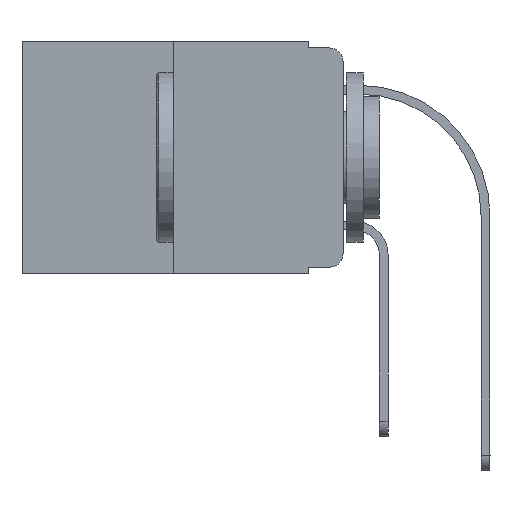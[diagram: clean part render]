
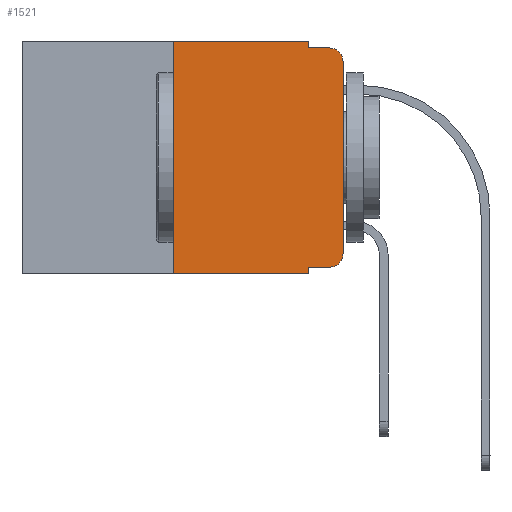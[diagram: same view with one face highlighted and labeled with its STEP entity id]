
A CAD part, left-side view. The second image highlights one B-rep face of the part: STEP entity #1521.
In plain terms, the highlighted planar face has unit normal (-1, 0, 0).
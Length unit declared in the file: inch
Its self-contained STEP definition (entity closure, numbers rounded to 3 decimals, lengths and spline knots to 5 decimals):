
#127 = ORIENTED_EDGE ( 'NONE', *, *, #3472, .F. ) ;
#410 = CARTESIAN_POINT ( 'NONE',  ( 0., 0.02, -0.313 ) ) ;
#486 = DIRECTION ( 'NONE',  ( 0., -1., 0. ) ) ;
#1039 = DIRECTION ( 'NONE',  ( 0., 0., 1. ) ) ;
#1069 = FACE_OUTER_BOUND ( 'NONE', #11055, .T. ) ;
#1080 = VERTEX_POINT ( 'NONE', #9564 ) ;
#1194 = DIRECTION ( 'NONE',  ( -1., 0., 0. ) ) ;
#1281 = CARTESIAN_POINT ( 'NONE',  ( 0., 0.25, 0. ) ) ;
#1407 = VECTOR ( 'NONE', #5567, 39.37008 ) ;
#1521 = ADVANCED_FACE ( 'NONE', ( #1069 ), #3092, .F. ) ;
#1807 = LINE ( 'NONE', #6082, #6714 ) ;
#1906 = CARTESIAN_POINT ( 'NONE',  ( 0., 0.02, -0.03 ) ) ;
#1920 = EDGE_CURVE ( 'NONE', #1080, #12006, #9822, .T. ) ;
#1961 = LINE ( 'NONE', #6384, #5870 ) ;
#2094 = LINE ( 'NONE', #6367, #11426 ) ;
#2271 = EDGE_CURVE ( 'NONE', #12852, #10443, #3841, .T. ) ;
#2323 = AXIS2_PLACEMENT_3D ( 'NONE', #410, #1194, #7557 ) ;
#2445 = VECTOR ( 'NONE', #7130, 39.37008 ) ;
#2518 = LINE ( 'NONE', #4681, #7609 ) ;
#2528 = CARTESIAN_POINT ( 'NONE',  ( 0., 0.051, 0. ) ) ;
#2994 = VERTEX_POINT ( 'NONE', #9002 ) ;
#3092 = PLANE ( 'NONE',  #12811 ) ;
#3226 = DIRECTION ( 'NONE',  ( -1., 0., 0. ) ) ;
#3443 = CARTESIAN_POINT ( 'NONE',  ( 0., 0.25, -0.343 ) ) ;
#3469 = LINE ( 'NONE', #11109, #1407 ) ;
#3472 = EDGE_CURVE ( 'NONE', #2994, #12006, #2518, .T. ) ;
#3476 = CARTESIAN_POINT ( 'NONE',  ( 0., 0.051, -0.333 ) ) ;
#3478 = ORIENTED_EDGE ( 'NONE', *, *, #9224, .F. ) ;
#3704 = CARTESIAN_POINT ( 'NONE',  ( 0., 0.051, -0.333 ) ) ;
#3841 = LINE ( 'NONE', #3704, #2445 ) ;
#3939 = CARTESIAN_POINT ( 'NONE',  ( 0., 0.051, 0. ) ) ;
#4446 = VERTEX_POINT ( 'NONE', #8286 ) ;
#4681 = CARTESIAN_POINT ( 'NONE',  ( 0., 0.051, -0.01 ) ) ;
#5018 = EDGE_CURVE ( 'NONE', #6952, #1080, #1961, .T. ) ;
#5145 = ORIENTED_EDGE ( 'NONE', *, *, #5708, .F. ) ;
#5567 = DIRECTION ( 'NONE',  ( 0., -1., 0. ) ) ;
#5659 = EDGE_CURVE ( 'NONE', #13784, #4446, #3469, .T. ) ;
#5668 = ORIENTED_EDGE ( 'NONE', *, *, #7876, .T. ) ;
#5708 = EDGE_CURVE ( 'NONE', #6629, #2994, #7042, .T. ) ;
#5870 = VECTOR ( 'NONE', #6236, 39.37008 ) ;
#5948 = DIRECTION ( 'NONE',  ( 0., -1., 0. ) ) ;
#5952 = CARTESIAN_POINT ( 'NONE',  ( 0., 0.051, 0. ) ) ;
#6082 = CARTESIAN_POINT ( 'NONE',  ( 0., 0.473, 0. ) ) ;
#6236 = DIRECTION ( 'NONE',  ( 0., 0., 1. ) ) ;
#6328 = VECTOR ( 'NONE', #8288, 39.37008 ) ;
#6367 = CARTESIAN_POINT ( 'NONE',  ( 0., 0.25, 0. ) ) ;
#6384 = CARTESIAN_POINT ( 'NONE',  ( 0., 0., 0. ) ) ;
#6424 = EDGE_CURVE ( 'NONE', #12852, #4446, #9957, .T. ) ;
#6629 = VERTEX_POINT ( 'NONE', #5952 ) ;
#6714 = VECTOR ( 'NONE', #486, 39.37008 ) ;
#6752 = ORIENTED_EDGE ( 'NONE', *, *, #1920, .T. ) ;
#6952 = VERTEX_POINT ( 'NONE', #7615 ) ;
#7042 = LINE ( 'NONE', #3939, #6328 ) ;
#7076 = ORIENTED_EDGE ( 'NONE', *, *, #2271, .T. ) ;
#7130 = DIRECTION ( 'NONE',  ( 0., -1., 0. ) ) ;
#7301 = CARTESIAN_POINT ( 'NONE',  ( 0., 0.473, 0. ) ) ;
#7557 = DIRECTION ( 'NONE',  ( 0., 0., -1. ) ) ;
#7609 = VECTOR ( 'NONE', #5948, 39.37008 ) ;
#7615 = CARTESIAN_POINT ( 'NONE',  ( 0., 0., -0.313 ) ) ;
#7625 = ORIENTED_EDGE ( 'NONE', *, *, #9437, .F. ) ;
#7876 = EDGE_CURVE ( 'NONE', #10443, #6952, #8354, .T. ) ;
#8286 = CARTESIAN_POINT ( 'NONE',  ( 0., 0.051, -0.343 ) ) ;
#8288 = DIRECTION ( 'NONE',  ( 0., 0., -1. ) ) ;
#8354 = CIRCLE ( 'NONE', #2323, 0.02 ) ;
#8576 = CARTESIAN_POINT ( 'NONE',  ( 0., 0.02, -0.333 ) ) ;
#8843 = ORIENTED_EDGE ( 'NONE', *, *, #5659, .T. ) ;
#9002 = CARTESIAN_POINT ( 'NONE',  ( 0., 0.051, -0.01 ) ) ;
#9224 = EDGE_CURVE ( 'NONE', #10415, #6629, #1807, .T. ) ;
#9437 = EDGE_CURVE ( 'NONE', #13784, #10415, #2094, .T. ) ;
#9551 = DIRECTION ( 'NONE',  ( 0., 0., -1. ) ) ;
#9564 = CARTESIAN_POINT ( 'NONE',  ( 0., 0., -0.03 ) ) ;
#9707 = VECTOR ( 'NONE', #9742, 39.37008 ) ;
#9742 = DIRECTION ( 'NONE',  ( 0., 0., -1. ) ) ;
#9822 = CIRCLE ( 'NONE', #10948, 0.02 ) ;
#9957 = LINE ( 'NONE', #2528, #9707 ) ;
#10281 = CARTESIAN_POINT ( 'NONE',  ( 0., 0.02, -0.01 ) ) ;
#10415 = VERTEX_POINT ( 'NONE', #1281 ) ;
#10443 = VERTEX_POINT ( 'NONE', #8576 ) ;
#10731 = DIRECTION ( 'NONE',  ( 1., 0., 0. ) ) ;
#10948 = AXIS2_PLACEMENT_3D ( 'NONE', #1906, #3226, #11634 ) ;
#11055 = EDGE_LOOP ( 'NONE', ( #13334, #6752, #127, #5145, #3478, #7625, #8843, #11763, #7076, #5668 ) ) ;
#11109 = CARTESIAN_POINT ( 'NONE',  ( 0., 0.473, -0.343 ) ) ;
#11426 = VECTOR ( 'NONE', #1039, 39.37008 ) ;
#11634 = DIRECTION ( 'NONE',  ( 0., 0., -1. ) ) ;
#11763 = ORIENTED_EDGE ( 'NONE', *, *, #6424, .F. ) ;
#12006 = VERTEX_POINT ( 'NONE', #10281 ) ;
#12811 = AXIS2_PLACEMENT_3D ( 'NONE', #7301, #10731, #9551 ) ;
#12852 = VERTEX_POINT ( 'NONE', #3476 ) ;
#13334 = ORIENTED_EDGE ( 'NONE', *, *, #5018, .T. ) ;
#13784 = VERTEX_POINT ( 'NONE', #3443 ) ;
